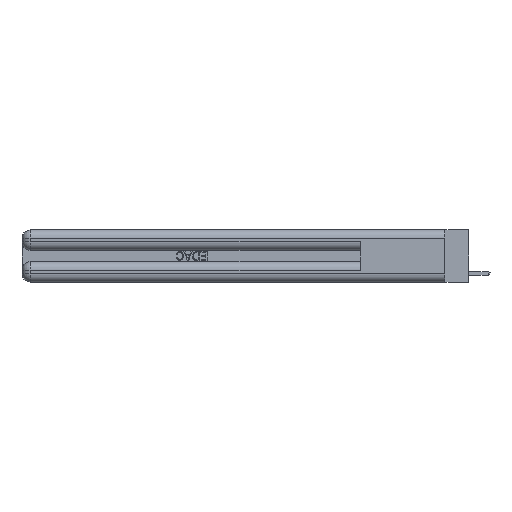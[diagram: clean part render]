
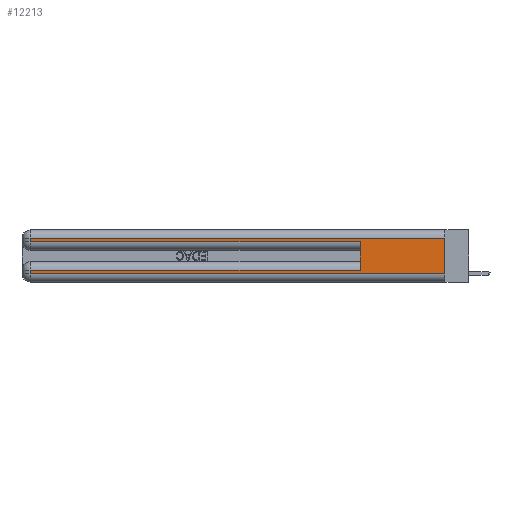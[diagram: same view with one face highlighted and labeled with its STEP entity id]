
A CAD part, left-side view. The second image highlights one B-rep face of the part: STEP entity #12213.
In plain terms, the highlighted planar face has unit normal (-1, 0, 0).
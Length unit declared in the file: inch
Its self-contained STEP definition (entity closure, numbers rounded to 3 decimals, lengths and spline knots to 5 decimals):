
#345 = DIRECTION ( 'NONE',  ( 0., 1., 0. ) ) ;
#1319 = DIRECTION ( 'NONE',  ( 0., 0., -1. ) ) ;
#1645 = CARTESIAN_POINT ( 'NONE',  ( 0., 0., 0.06 ) ) ;
#2194 = CARTESIAN_POINT ( 'NONE',  ( 0., 0.6, 0.285 ) ) ;
#2477 = VECTOR ( 'NONE', #4635, 39.37008 ) ;
#3231 = LINE ( 'NONE', #13779, #5409 ) ;
#3937 = LINE ( 'NONE', #25084, #2477 ) ;
#4635 = DIRECTION ( 'NONE',  ( 0., 0., -1. ) ) ;
#5221 = DIRECTION ( 'NONE',  ( 1., 0., 0. ) ) ;
#5403 = VERTEX_POINT ( 'NONE', #13728 ) ;
#5409 = VECTOR ( 'NONE', #11876, 39.37008 ) ;
#5718 = DIRECTION ( 'NONE',  ( 0., 0., -1. ) ) ;
#6303 = DIRECTION ( 'NONE',  ( 0., 1., 0. ) ) ;
#6790 = EDGE_CURVE ( 'NONE', #18068, #28766, #24730, .T. ) ;
#7180 = DIRECTION ( 'NONE',  ( 0., -1., 0. ) ) ;
#7437 = ORIENTED_EDGE ( 'NONE', *, *, #13575, .F. ) ;
#7464 = EDGE_CURVE ( 'NONE', #18068, #18201, #26691, .T. ) ;
#8741 = ORIENTED_EDGE ( 'NONE', *, *, #14091, .T. ) ;
#9287 = CARTESIAN_POINT ( 'NONE',  ( 0., 2.94, 0.31 ) ) ;
#9565 = VECTOR ( 'NONE', #7180, 39.37008 ) ;
#9620 = EDGE_CURVE ( 'NONE', #5403, #15995, #15265, .T. ) ;
#10007 = ORIENTED_EDGE ( 'NONE', *, *, #7464, .T. ) ;
#10456 = EDGE_CURVE ( 'NONE', #15995, #19416, #3937, .T. ) ;
#10574 = DIRECTION ( 'NONE',  ( 0., 0., 1. ) ) ;
#11071 = ORIENTED_EDGE ( 'NONE', *, *, #10456, .T. ) ;
#11378 = VECTOR ( 'NONE', #11531, 39.37008 ) ;
#11531 = DIRECTION ( 'NONE',  ( 0., 0., -1. ) ) ;
#11681 = VECTOR ( 'NONE', #1319, 39.37008 ) ;
#11876 = DIRECTION ( 'NONE',  ( 0., -1., 0. ) ) ;
#12213 = ADVANCED_FACE ( 'NONE', ( #21681 ), #13499, .F. ) ;
#12228 = CARTESIAN_POINT ( 'NONE',  ( 0., 2.94, 0.06 ) ) ;
#13499 = PLANE ( 'NONE',  #13540 ) ;
#13540 = AXIS2_PLACEMENT_3D ( 'NONE', #26533, #5221, #5718 ) ;
#13575 = EDGE_CURVE ( 'NONE', #5403, #32417, #24448, .T. ) ;
#13670 = CARTESIAN_POINT ( 'NONE',  ( 0., 0.6, 0.145 ) ) ;
#13728 = CARTESIAN_POINT ( 'NONE',  ( 0., 0.6, 0.085 ) ) ;
#13779 = CARTESIAN_POINT ( 'NONE',  ( 0., 0., 0.285 ) ) ;
#14023 = CARTESIAN_POINT ( 'NONE',  ( 0., 2.94, 0.285 ) ) ;
#14091 = EDGE_CURVE ( 'NONE', #18201, #15814, #14670, .T. ) ;
#14670 = LINE ( 'NONE', #25273, #11378 ) ;
#15265 = LINE ( 'NONE', #25213, #24052 ) ;
#15814 = VERTEX_POINT ( 'NONE', #14023 ) ;
#15995 = VERTEX_POINT ( 'NONE', #22905 ) ;
#17866 = VECTOR ( 'NONE', #345, 39.37008 ) ;
#18068 = VERTEX_POINT ( 'NONE', #32347 ) ;
#18201 = VERTEX_POINT ( 'NONE', #9287 ) ;
#19416 = VERTEX_POINT ( 'NONE', #12228 ) ;
#20428 = ORIENTED_EDGE ( 'NONE', *, *, #6790, .F. ) ;
#20900 = LINE ( 'NONE', #1645, #9565 ) ;
#21681 = FACE_OUTER_BOUND ( 'NONE', #22297, .T. ) ;
#22297 = EDGE_LOOP ( 'NONE', ( #20428, #10007, #8741, #22798, #7437, #23224, #11071, #34245 ) ) ;
#22798 = ORIENTED_EDGE ( 'NONE', *, *, #30697, .T. ) ;
#22905 = CARTESIAN_POINT ( 'NONE',  ( 0., 2.94, 0.085 ) ) ;
#23224 = ORIENTED_EDGE ( 'NONE', *, *, #9620, .T. ) ;
#23360 = EDGE_CURVE ( 'NONE', #19416, #28766, #20900, .T. ) ;
#24052 = VECTOR ( 'NONE', #6303, 39.37008 ) ;
#24448 = LINE ( 'NONE', #13670, #30772 ) ;
#24730 = LINE ( 'NONE', #25071, #11681 ) ;
#25071 = CARTESIAN_POINT ( 'NONE',  ( 0., 0., 0.37 ) ) ;
#25084 = CARTESIAN_POINT ( 'NONE',  ( 0., 2.94, 0.37 ) ) ;
#25213 = CARTESIAN_POINT ( 'NONE',  ( 0., 0., 0.085 ) ) ;
#25273 = CARTESIAN_POINT ( 'NONE',  ( 0., 2.94, 0.37 ) ) ;
#26533 = CARTESIAN_POINT ( 'NONE',  ( 0., 0., 0.37 ) ) ;
#26691 = LINE ( 'NONE', #29467, #17866 ) ;
#28766 = VERTEX_POINT ( 'NONE', #33650 ) ;
#29467 = CARTESIAN_POINT ( 'NONE',  ( 0., 0., 0.31 ) ) ;
#30697 = EDGE_CURVE ( 'NONE', #15814, #32417, #3231, .T. ) ;
#30772 = VECTOR ( 'NONE', #10574, 39.37008 ) ;
#32347 = CARTESIAN_POINT ( 'NONE',  ( 0., 0., 0.31 ) ) ;
#32417 = VERTEX_POINT ( 'NONE', #2194 ) ;
#33650 = CARTESIAN_POINT ( 'NONE',  ( 0., 0., 0.06 ) ) ;
#34245 = ORIENTED_EDGE ( 'NONE', *, *, #23360, .T. ) ;
